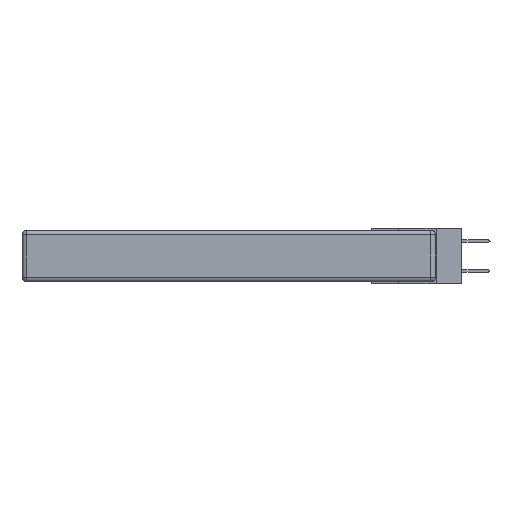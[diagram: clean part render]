
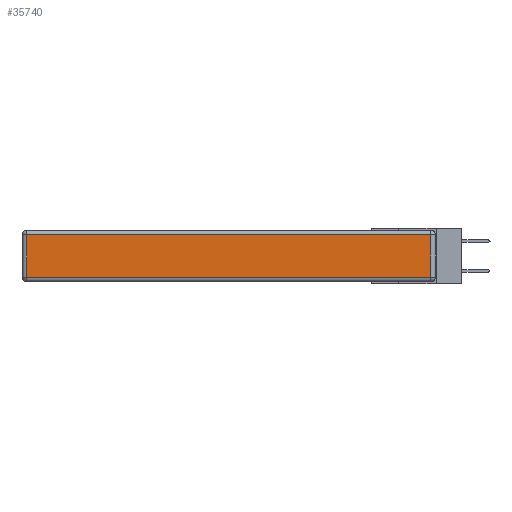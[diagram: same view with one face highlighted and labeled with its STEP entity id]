
A CAD part, left-side view. The second image highlights one B-rep face of the part: STEP entity #35740.
In plain terms, the highlighted planar face has unit normal (-1, 0, 0).
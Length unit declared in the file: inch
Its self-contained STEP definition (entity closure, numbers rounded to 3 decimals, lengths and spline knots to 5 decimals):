
#1382 = EDGE_CURVE ( 'NONE', #12667, #31833, #15505, .T. ) ;
#2253 = VERTEX_POINT ( 'NONE', #11717 ) ;
#2333 = CARTESIAN_POINT ( 'NONE',  ( 0., 2.72, -0.313 ) ) ;
#3210 = EDGE_LOOP ( 'NONE', ( #8766, #11182, #19755, #22318 ) ) ;
#5709 = VERTEX_POINT ( 'NONE', #2333 ) ;
#6325 = EDGE_CURVE ( 'NONE', #5709, #2253, #10272, .T. ) ;
#6706 = VECTOR ( 'NONE', #8518, 39.37008 ) ;
#7589 = CARTESIAN_POINT ( 'NONE',  ( 0., 0., -0.343 ) ) ;
#8230 = DIRECTION ( 'NONE',  ( 0., 0., -1. ) ) ;
#8518 = DIRECTION ( 'NONE',  ( 0., 1., 0. ) ) ;
#8766 = ORIENTED_EDGE ( 'NONE', *, *, #6325, .T. ) ;
#9270 = FACE_OUTER_BOUND ( 'NONE', #3210, .T. ) ;
#10272 = LINE ( 'NONE', #28998, #18174 ) ;
#11182 = ORIENTED_EDGE ( 'NONE', *, *, #24143, .T. ) ;
#11717 = CARTESIAN_POINT ( 'NONE',  ( 0., 0.03, -0.313 ) ) ;
#11986 = DIRECTION ( 'NONE',  ( 0., 0., 1. ) ) ;
#12667 = VERTEX_POINT ( 'NONE', #32803 ) ;
#13617 = CARTESIAN_POINT ( 'NONE',  ( 0., 2.72, -0.343 ) ) ;
#15505 = LINE ( 'NONE', #24961, #6706 ) ;
#15592 = VECTOR ( 'NONE', #8230, 39.37008 ) ;
#18174 = VECTOR ( 'NONE', #23252, 39.37008 ) ;
#19072 = CARTESIAN_POINT ( 'NONE',  ( 0., 2.72, -0.03 ) ) ;
#19383 = VECTOR ( 'NONE', #11986, 39.37008 ) ;
#19755 = ORIENTED_EDGE ( 'NONE', *, *, #1382, .T. ) ;
#21130 = EDGE_CURVE ( 'NONE', #31833, #5709, #33987, .T. ) ;
#22318 = ORIENTED_EDGE ( 'NONE', *, *, #21130, .T. ) ;
#22409 = DIRECTION ( 'NONE',  ( 0., 0., 1. ) ) ;
#23252 = DIRECTION ( 'NONE',  ( 0., -1., 0. ) ) ;
#24143 = EDGE_CURVE ( 'NONE', #2253, #12667, #26817, .T. ) ;
#24391 = PLANE ( 'NONE',  #33132 ) ;
#24961 = CARTESIAN_POINT ( 'NONE',  ( 0., 2.75, -0.03 ) ) ;
#26817 = LINE ( 'NONE', #31807, #19383 ) ;
#28998 = CARTESIAN_POINT ( 'NONE',  ( 0., 0., -0.313 ) ) ;
#31807 = CARTESIAN_POINT ( 'NONE',  ( 0., 0.03, -0.343 ) ) ;
#31833 = VERTEX_POINT ( 'NONE', #19072 ) ;
#32803 = CARTESIAN_POINT ( 'NONE',  ( 0., 0.03, -0.03 ) ) ;
#33132 = AXIS2_PLACEMENT_3D ( 'NONE', #7589, #33277, #22409 ) ;
#33277 = DIRECTION ( 'NONE',  ( -1., 0., 0. ) ) ;
#33987 = LINE ( 'NONE', #13617, #15592 ) ;
#35740 = ADVANCED_FACE ( 'NONE', ( #9270 ), #24391, .T. ) ;
